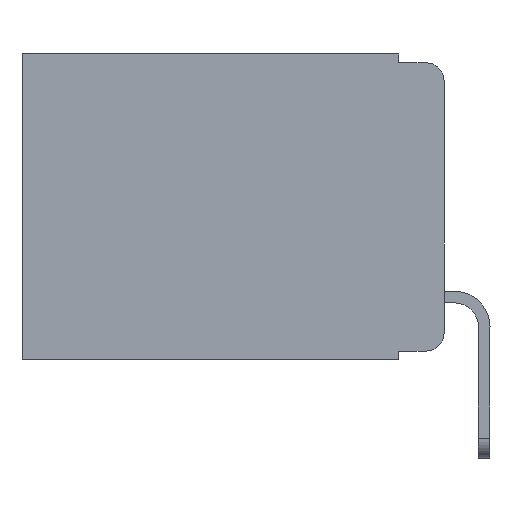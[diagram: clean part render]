
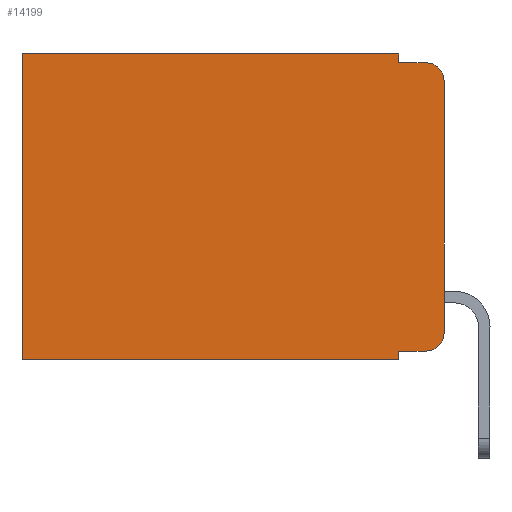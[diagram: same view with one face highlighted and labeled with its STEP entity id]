
A CAD part, left-side view. The second image highlights one B-rep face of the part: STEP entity #14199.
In plain terms, the highlighted planar face has unit normal (-1, 0, 0).
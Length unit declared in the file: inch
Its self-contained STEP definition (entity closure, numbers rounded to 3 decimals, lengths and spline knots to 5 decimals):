
#156 = DIRECTION ( 'NONE',  ( 0., -1., 0. ) ) ;
#157 = VERTEX_POINT ( 'NONE', #15516 ) ;
#276 = CARTESIAN_POINT ( 'NONE',  ( 0.298, 0.051, -0.01 ) ) ;
#454 = EDGE_LOOP ( 'NONE', ( #10101, #11615, #7112, #6422, #16295, #16775, #8428, #14568, #13032, #7514 ) ) ;
#629 = DIRECTION ( 'NONE',  ( 0., 1., 0. ) ) ;
#1073 = CARTESIAN_POINT ( 'NONE',  ( 0.298, 0., -0.343 ) ) ;
#1215 = CARTESIAN_POINT ( 'NONE',  ( 0.298, 0.051, -0.333 ) ) ;
#1224 = CARTESIAN_POINT ( 'NONE',  ( 0.298, 0., -0.03 ) ) ;
#1497 = EDGE_CURVE ( 'NONE', #10464, #157, #13310, .T. ) ;
#1967 = CARTESIAN_POINT ( 'NONE',  ( 0.298, 0.473, 0. ) ) ;
#2421 = CARTESIAN_POINT ( 'NONE',  ( 0.298, 0.02, -0.03 ) ) ;
#2473 = VECTOR ( 'NONE', #10583, 39.37008 ) ;
#2480 = LINE ( 'NONE', #12577, #9681 ) ;
#2645 = VERTEX_POINT ( 'NONE', #3758 ) ;
#3280 = CARTESIAN_POINT ( 'NONE',  ( 0.298, 0., 0. ) ) ;
#3629 = CIRCLE ( 'NONE', #16778, 0.02 ) ;
#3642 = DIRECTION ( 'NONE',  ( 0., 0., -1. ) ) ;
#3758 = CARTESIAN_POINT ( 'NONE',  ( 0.298, 0.051, -0.343 ) ) ;
#4032 = CARTESIAN_POINT ( 'NONE',  ( 0.298, 0.02, -0.333 ) ) ;
#4187 = CARTESIAN_POINT ( 'NONE',  ( 0.298, 0.02, -0.313 ) ) ;
#5270 = EDGE_CURVE ( 'NONE', #10160, #13836, #14638, .T. ) ;
#5796 = DIRECTION ( 'NONE',  ( 0., -1., 0. ) ) ;
#6299 = FACE_OUTER_BOUND ( 'NONE', #454, .T. ) ;
#6422 = ORIENTED_EDGE ( 'NONE', *, *, #1497, .F. ) ;
#6423 = CARTESIAN_POINT ( 'NONE',  ( 0.298, 0.051, 0. ) ) ;
#6434 = EDGE_CURVE ( 'NONE', #14636, #7476, #6868, .T. ) ;
#6533 = DIRECTION ( 'NONE',  ( 0., 0., -1. ) ) ;
#6574 = LINE ( 'NONE', #15820, #7414 ) ;
#6848 = DIRECTION ( 'NONE',  ( 0., 0., -1. ) ) ;
#6857 = LINE ( 'NONE', #13045, #14500 ) ;
#6868 = CIRCLE ( 'NONE', #13870, 0.02 ) ;
#6968 = LINE ( 'NONE', #3280, #9521 ) ;
#7112 = ORIENTED_EDGE ( 'NONE', *, *, #8722, .F. ) ;
#7414 = VECTOR ( 'NONE', #6533, 39.37008 ) ;
#7476 = VERTEX_POINT ( 'NONE', #9124 ) ;
#7514 = ORIENTED_EDGE ( 'NONE', *, *, #6434, .T. ) ;
#7601 = DIRECTION ( 'NONE',  ( 0., 1., 0. ) ) ;
#7945 = EDGE_CURVE ( 'NONE', #9946, #7476, #6574, .T. ) ;
#8022 = EDGE_CURVE ( 'NONE', #9946, #17466, #3629, .T. ) ;
#8428 = ORIENTED_EDGE ( 'NONE', *, *, #11818, .F. ) ;
#8722 = EDGE_CURVE ( 'NONE', #157, #17466, #15689, .T. ) ;
#8773 = DIRECTION ( 'NONE',  ( 1., 0., 0. ) ) ;
#8854 = CARTESIAN_POINT ( 'NONE',  ( 0.298, 0.473, -0.343 ) ) ;
#9124 = CARTESIAN_POINT ( 'NONE',  ( 0.298, 0., -0.313 ) ) ;
#9334 = LINE ( 'NONE', #1073, #15279 ) ;
#9521 = VECTOR ( 'NONE', #629, 39.37008 ) ;
#9681 = VECTOR ( 'NONE', #5796, 39.37008 ) ;
#9946 = VERTEX_POINT ( 'NONE', #1224 ) ;
#10101 = ORIENTED_EDGE ( 'NONE', *, *, #7945, .F. ) ;
#10160 = VERTEX_POINT ( 'NONE', #1967 ) ;
#10464 = VERTEX_POINT ( 'NONE', #10485 ) ;
#10485 = CARTESIAN_POINT ( 'NONE',  ( 0.298, 0.051, 0. ) ) ;
#10583 = DIRECTION ( 'NONE',  ( 0., 0., -1. ) ) ;
#10901 = DIRECTION ( 'NONE',  ( 0., 0., -1. ) ) ;
#10990 = EDGE_CURVE ( 'NONE', #15123, #14636, #2480, .T. ) ;
#11054 = VECTOR ( 'NONE', #10901, 39.37008 ) ;
#11121 = AXIS2_PLACEMENT_3D ( 'NONE', #16864, #8773, #17011 ) ;
#11562 = DIRECTION ( 'NONE',  ( 0., 0., -1. ) ) ;
#11615 = ORIENTED_EDGE ( 'NONE', *, *, #8022, .T. ) ;
#11818 = EDGE_CURVE ( 'NONE', #2645, #13836, #9334, .T. ) ;
#12134 = VECTOR ( 'NONE', #156, 39.37008 ) ;
#12577 = CARTESIAN_POINT ( 'NONE',  ( 0.298, 0.051, -0.333 ) ) ;
#12773 = PLANE ( 'NONE',  #11121 ) ;
#12813 = EDGE_CURVE ( 'NONE', #10464, #10160, #6968, .T. ) ;
#13032 = ORIENTED_EDGE ( 'NONE', *, *, #10990, .T. ) ;
#13045 = CARTESIAN_POINT ( 'NONE',  ( 0.298, 0.051, 0. ) ) ;
#13310 = LINE ( 'NONE', #6423, #2473 ) ;
#13836 = VERTEX_POINT ( 'NONE', #8854 ) ;
#13870 = AXIS2_PLACEMENT_3D ( 'NONE', #4187, #15161, #6848 ) ;
#14199 = ADVANCED_FACE ( 'NONE', ( #6299 ), #12773, .F. ) ;
#14500 = VECTOR ( 'NONE', #11562, 39.37008 ) ;
#14568 = ORIENTED_EDGE ( 'NONE', *, *, #16254, .F. ) ;
#14636 = VERTEX_POINT ( 'NONE', #4032 ) ;
#14638 = LINE ( 'NONE', #16187, #11054 ) ;
#15123 = VERTEX_POINT ( 'NONE', #1215 ) ;
#15161 = DIRECTION ( 'NONE',  ( -1., 0., 0. ) ) ;
#15279 = VECTOR ( 'NONE', #7601, 39.37008 ) ;
#15444 = CARTESIAN_POINT ( 'NONE',  ( 0.298, 0.02, -0.01 ) ) ;
#15516 = CARTESIAN_POINT ( 'NONE',  ( 0.298, 0.051, -0.01 ) ) ;
#15689 = LINE ( 'NONE', #276, #12134 ) ;
#15763 = DIRECTION ( 'NONE',  ( -1., 0., 0. ) ) ;
#15820 = CARTESIAN_POINT ( 'NONE',  ( 0.298, 0., 0. ) ) ;
#16187 = CARTESIAN_POINT ( 'NONE',  ( 0.298, 0.473, 0. ) ) ;
#16254 = EDGE_CURVE ( 'NONE', #15123, #2645, #6857, .T. ) ;
#16295 = ORIENTED_EDGE ( 'NONE', *, *, #12813, .T. ) ;
#16775 = ORIENTED_EDGE ( 'NONE', *, *, #5270, .T. ) ;
#16778 = AXIS2_PLACEMENT_3D ( 'NONE', #2421, #15763, #3642 ) ;
#16864 = CARTESIAN_POINT ( 'NONE',  ( 0.298, 0., 0. ) ) ;
#17011 = DIRECTION ( 'NONE',  ( 0., 0., -1. ) ) ;
#17466 = VERTEX_POINT ( 'NONE', #15444 ) ;
